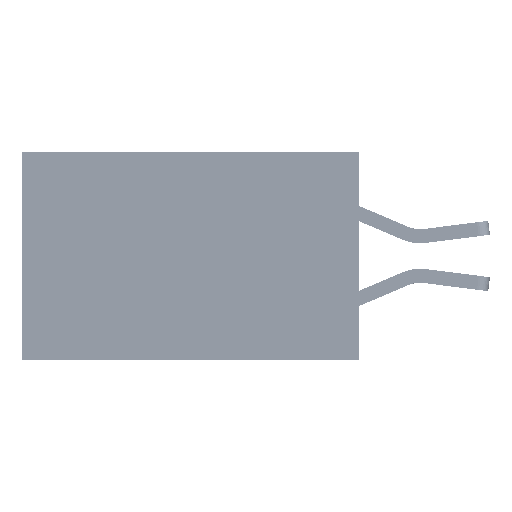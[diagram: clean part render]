
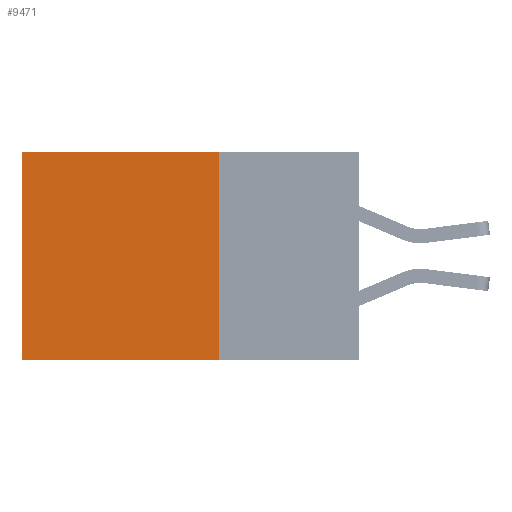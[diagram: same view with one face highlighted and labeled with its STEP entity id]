
A CAD part, left-side view. The second image highlights one B-rep face of the part: STEP entity #9471.
In plain terms, the highlighted planar face has unit normal (-1, 0, 0).
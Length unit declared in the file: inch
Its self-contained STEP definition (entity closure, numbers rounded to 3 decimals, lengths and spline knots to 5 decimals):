
#340 = LINE ( 'NONE', #35773, #34571 ) ;
#799 = VECTOR ( 'NONE', #19529, 39.37008 ) ;
#1021 = VERTEX_POINT ( 'NONE', #34137 ) ;
#1194 = CARTESIAN_POINT ( 'NONE',  ( 0.2875, 0.6, -0.37 ) ) ;
#3073 = CARTESIAN_POINT ( 'NONE',  ( 0.2875, 0.25, 0. ) ) ;
#6177 = VERTEX_POINT ( 'NONE', #33886 ) ;
#6883 = EDGE_CURVE ( 'NONE', #6177, #17128, #14866, .T. ) ;
#8977 = EDGE_CURVE ( 'NONE', #6177, #1021, #15767, .T. ) ;
#9471 = ADVANCED_FACE ( 'NONE', ( #28958 ), #12878, .F. ) ;
#10472 = VERTEX_POINT ( 'NONE', #1194 ) ;
#10711 = EDGE_LOOP ( 'NONE', ( #37659, #36371, #22224, #36546 ) ) ;
#12878 = PLANE ( 'NONE',  #21621 ) ;
#13618 = DIRECTION ( 'NONE',  ( 0., 0., -1. ) ) ;
#14866 = LINE ( 'NONE', #16704, #799 ) ;
#15767 = LINE ( 'NONE', #3073, #35460 ) ;
#16704 = CARTESIAN_POINT ( 'NONE',  ( 0.2875, 0.25, 0. ) ) ;
#17128 = VERTEX_POINT ( 'NONE', #19043 ) ;
#17694 = DIRECTION ( 'NONE',  ( 0., 1., 0. ) ) ;
#18763 = CARTESIAN_POINT ( 'NONE',  ( 0.2875, 0.25, 0. ) ) ;
#18855 = EDGE_CURVE ( 'NONE', #17128, #10472, #28191, .T. ) ;
#19043 = CARTESIAN_POINT ( 'NONE',  ( 0.2875, 0.25, -0.37 ) ) ;
#19529 = DIRECTION ( 'NONE',  ( 0., 0., -1. ) ) ;
#19545 = EDGE_CURVE ( 'NONE', #1021, #10472, #340, .T. ) ;
#21621 = AXIS2_PLACEMENT_3D ( 'NONE', #18763, #35918, #13618 ) ;
#22224 = ORIENTED_EDGE ( 'NONE', *, *, #6883, .F. ) ;
#27757 = VECTOR ( 'NONE', #36431, 39.37008 ) ;
#28191 = LINE ( 'NONE', #36687, #27757 ) ;
#28958 = FACE_OUTER_BOUND ( 'NONE', #10711, .T. ) ;
#32965 = DIRECTION ( 'NONE',  ( 0., 0., -1. ) ) ;
#33886 = CARTESIAN_POINT ( 'NONE',  ( 0.2875, 0.25, 0. ) ) ;
#34137 = CARTESIAN_POINT ( 'NONE',  ( 0.2875, 0.6, 0. ) ) ;
#34571 = VECTOR ( 'NONE', #32965, 39.37008 ) ;
#35460 = VECTOR ( 'NONE', #17694, 39.37008 ) ;
#35773 = CARTESIAN_POINT ( 'NONE',  ( 0.2875, 0.6, 0. ) ) ;
#35918 = DIRECTION ( 'NONE',  ( 1., 0., 0. ) ) ;
#36371 = ORIENTED_EDGE ( 'NONE', *, *, #18855, .F. ) ;
#36431 = DIRECTION ( 'NONE',  ( 0., 1., 0. ) ) ;
#36546 = ORIENTED_EDGE ( 'NONE', *, *, #8977, .T. ) ;
#36687 = CARTESIAN_POINT ( 'NONE',  ( 0.2875, 0.25, -0.37 ) ) ;
#37659 = ORIENTED_EDGE ( 'NONE', *, *, #19545, .T. ) ;
